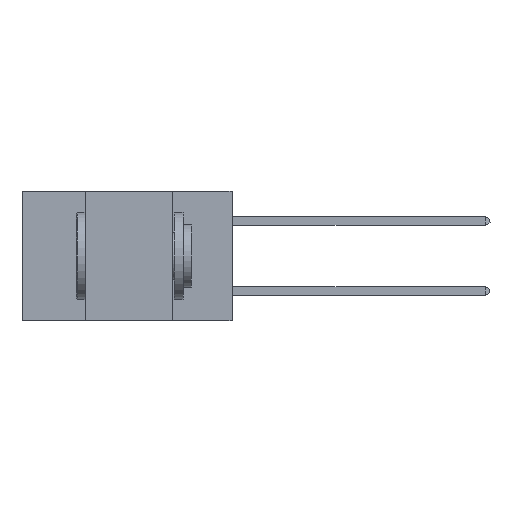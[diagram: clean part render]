
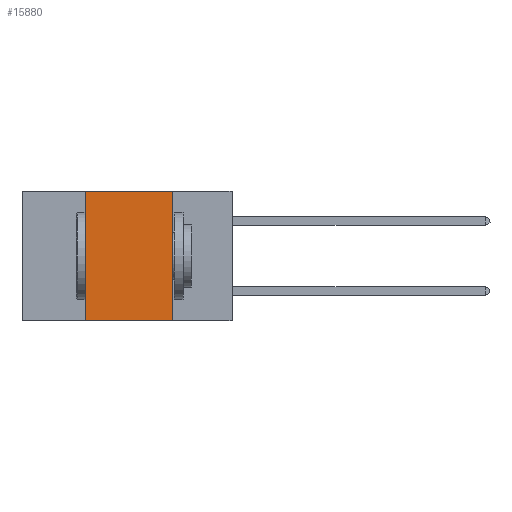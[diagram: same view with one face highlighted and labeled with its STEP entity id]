
A CAD part, left-side view. The second image highlights one B-rep face of the part: STEP entity #15880.
In plain terms, the highlighted planar face has unit normal (-1, 0, 0).
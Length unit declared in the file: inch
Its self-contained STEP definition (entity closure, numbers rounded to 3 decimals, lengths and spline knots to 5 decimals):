
#236 = DIRECTION ( 'NONE',  ( 0., 0., -1. ) ) ;
#931 = AXIS2_PLACEMENT_3D ( 'NONE', #21592, #14520, #4109 ) ;
#1476 = EDGE_LOOP ( 'NONE', ( #15060, #17942, #12514, #5169 ) ) ;
#2734 = LINE ( 'NONE', #10635, #16022 ) ;
#3085 = VECTOR ( 'NONE', #20641, 39.37008 ) ;
#3396 = VECTOR ( 'NONE', #17632, 39.37008 ) ;
#4109 = DIRECTION ( 'NONE',  ( 0., 0., -1. ) ) ;
#4290 = DIRECTION ( 'NONE',  ( 0., -1., 0. ) ) ;
#4513 = CARTESIAN_POINT ( 'NONE',  ( 0., 0.17, 0. ) ) ;
#5143 = CARTESIAN_POINT ( 'NONE',  ( 0., 0.42, 0. ) ) ;
#5169 = ORIENTED_EDGE ( 'NONE', *, *, #9129, .T. ) ;
#5871 = CARTESIAN_POINT ( 'NONE',  ( 0., 0.42, -0.37 ) ) ;
#7327 = VECTOR ( 'NONE', #4290, 39.37008 ) ;
#8085 = VERTEX_POINT ( 'NONE', #14934 ) ;
#8981 = CARTESIAN_POINT ( 'NONE',  ( 0., 0.17, -0.37 ) ) ;
#9129 = EDGE_CURVE ( 'NONE', #13648, #13419, #17768, .T. ) ;
#10635 = CARTESIAN_POINT ( 'NONE',  ( 0., 0.17, 0. ) ) ;
#12397 = EDGE_CURVE ( 'NONE', #8085, #13413, #14122, .T. ) ;
#12514 = ORIENTED_EDGE ( 'NONE', *, *, #18177, .F. ) ;
#13413 = VERTEX_POINT ( 'NONE', #4513 ) ;
#13419 = VERTEX_POINT ( 'NONE', #8981 ) ;
#13648 = VERTEX_POINT ( 'NONE', #5871 ) ;
#14122 = LINE ( 'NONE', #17356, #7327 ) ;
#14449 = LINE ( 'NONE', #5143, #3085 ) ;
#14520 = DIRECTION ( 'NONE',  ( 1., 0., 0. ) ) ;
#14934 = CARTESIAN_POINT ( 'NONE',  ( 0., 0.42, 0. ) ) ;
#15060 = ORIENTED_EDGE ( 'NONE', *, *, #19096, .F. ) ;
#15682 = CARTESIAN_POINT ( 'NONE',  ( 0., 0.6, -0.37 ) ) ;
#15880 = ADVANCED_FACE ( 'NONE', ( #19164 ), #19848, .F. ) ;
#16022 = VECTOR ( 'NONE', #236, 39.37008 ) ;
#17356 = CARTESIAN_POINT ( 'NONE',  ( 0., 0.6, 0. ) ) ;
#17632 = DIRECTION ( 'NONE',  ( 0., -1., 0. ) ) ;
#17768 = LINE ( 'NONE', #15682, #3396 ) ;
#17942 = ORIENTED_EDGE ( 'NONE', *, *, #12397, .F. ) ;
#18177 = EDGE_CURVE ( 'NONE', #13648, #8085, #14449, .T. ) ;
#19096 = EDGE_CURVE ( 'NONE', #13413, #13419, #2734, .T. ) ;
#19164 = FACE_OUTER_BOUND ( 'NONE', #1476, .T. ) ;
#19848 = PLANE ( 'NONE',  #931 ) ;
#20641 = DIRECTION ( 'NONE',  ( 0., 0., 1. ) ) ;
#21592 = CARTESIAN_POINT ( 'NONE',  ( 0., 0.6, 0. ) ) ;
